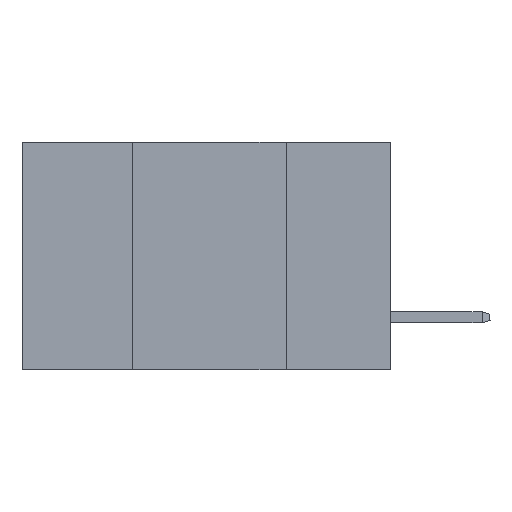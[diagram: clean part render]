
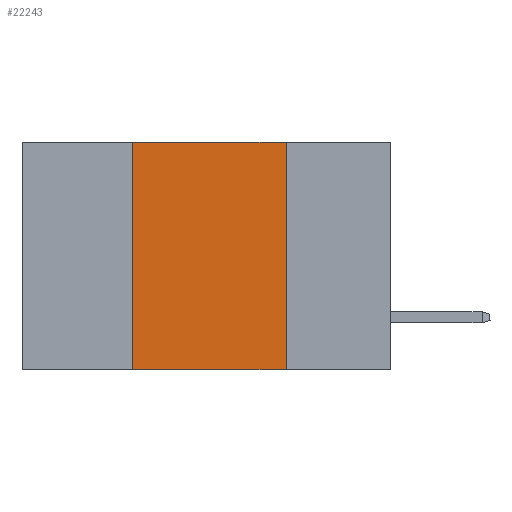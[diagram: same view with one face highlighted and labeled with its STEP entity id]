
A CAD part, left-side view. The second image highlights one B-rep face of the part: STEP entity #22243.
In plain terms, the highlighted planar face has unit normal (-1, 0, 0).
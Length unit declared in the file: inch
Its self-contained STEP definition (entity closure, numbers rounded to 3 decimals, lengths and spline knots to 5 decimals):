
#258 = VERTEX_POINT ( 'NONE', #21738 ) ;
#1492 = CARTESIAN_POINT ( 'NONE',  ( 0., 0.17, 0. ) ) ;
#3673 = DIRECTION ( 'NONE',  ( 0., -1., 0. ) ) ;
#3988 = DIRECTION ( 'NONE',  ( 0., -1., 0. ) ) ;
#5513 = VECTOR ( 'NONE', #27408, 39.37008 ) ;
#6667 = DIRECTION ( 'NONE',  ( 0., 0., -1. ) ) ;
#8839 = CARTESIAN_POINT ( 'NONE',  ( 0., 0.42, 0. ) ) ;
#8865 = CARTESIAN_POINT ( 'NONE',  ( 0., 0.6, 0. ) ) ;
#9102 = FACE_OUTER_BOUND ( 'NONE', #30381, .T. ) ;
#10146 = VERTEX_POINT ( 'NONE', #11296 ) ;
#10194 = EDGE_CURVE ( 'NONE', #14615, #10146, #22508, .T. ) ;
#10320 = ORIENTED_EDGE ( 'NONE', *, *, #10194, .F. ) ;
#11184 = VECTOR ( 'NONE', #3988, 39.37008 ) ;
#11296 = CARTESIAN_POINT ( 'NONE',  ( 0., 0.17, -0.37 ) ) ;
#11672 = DIRECTION ( 'NONE',  ( 1., 0., 0. ) ) ;
#12918 = LINE ( 'NONE', #27944, #11184 ) ;
#14615 = VERTEX_POINT ( 'NONE', #1492 ) ;
#14618 = CARTESIAN_POINT ( 'NONE',  ( 0., 0.6, 0. ) ) ;
#16810 = CARTESIAN_POINT ( 'NONE',  ( 0., 0.17, 0. ) ) ;
#17714 = EDGE_CURVE ( 'NONE', #29505, #14615, #25201, .T. ) ;
#21738 = CARTESIAN_POINT ( 'NONE',  ( 0., 0.42, -0.37 ) ) ;
#22243 = ADVANCED_FACE ( 'NONE', ( #9102 ), #33168, .F. ) ;
#22508 = LINE ( 'NONE', #16810, #5513 ) ;
#24021 = ORIENTED_EDGE ( 'NONE', *, *, #17714, .F. ) ;
#24322 = AXIS2_PLACEMENT_3D ( 'NONE', #14618, #11672, #6667 ) ;
#24465 = DIRECTION ( 'NONE',  ( 0., 0., 1. ) ) ;
#24839 = ORIENTED_EDGE ( 'NONE', *, *, #28668, .F. ) ;
#24913 = EDGE_CURVE ( 'NONE', #258, #10146, #12918, .T. ) ;
#25201 = LINE ( 'NONE', #8865, #30127 ) ;
#25507 = VECTOR ( 'NONE', #24465, 39.37008 ) ;
#27408 = DIRECTION ( 'NONE',  ( 0., 0., -1. ) ) ;
#27944 = CARTESIAN_POINT ( 'NONE',  ( 0., 0.6, -0.37 ) ) ;
#28575 = ORIENTED_EDGE ( 'NONE', *, *, #24913, .T. ) ;
#28668 = EDGE_CURVE ( 'NONE', #258, #29505, #30843, .T. ) ;
#29505 = VERTEX_POINT ( 'NONE', #30910 ) ;
#30127 = VECTOR ( 'NONE', #3673, 39.37008 ) ;
#30381 = EDGE_LOOP ( 'NONE', ( #10320, #24021, #24839, #28575 ) ) ;
#30843 = LINE ( 'NONE', #8839, #25507 ) ;
#30910 = CARTESIAN_POINT ( 'NONE',  ( 0., 0.42, 0. ) ) ;
#33168 = PLANE ( 'NONE',  #24322 ) ;
